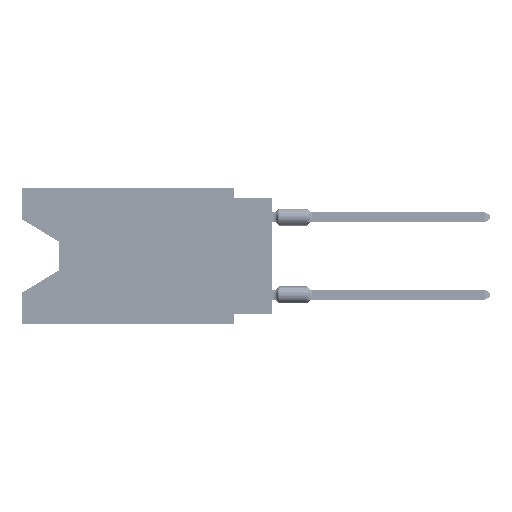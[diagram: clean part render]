
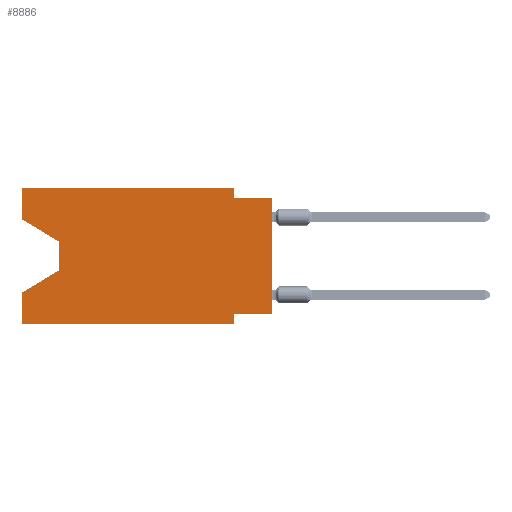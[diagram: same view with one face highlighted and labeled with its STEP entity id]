
A CAD part, left-side view. The second image highlights one B-rep face of the part: STEP entity #8886.
In plain terms, the highlighted planar face has unit normal (-1, 0, 0).
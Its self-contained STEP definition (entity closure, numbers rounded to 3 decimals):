
#264 = ORIENTED_EDGE ( 'NONE', *, *, #69302, .F. ) ;
#595 = CARTESIAN_POINT ( 'NONE',  ( 0., 13.97, -5.385 ) ) ;
#1083 = VERTEX_POINT ( 'NONE', #35631 ) ;
#1825 = VERTEX_POINT ( 'NONE', #34298 ) ;
#2641 = VERTEX_POINT ( 'NONE', #7301 ) ;
#3110 = LINE ( 'NONE', #29963, #32450 ) ;
#3960 = CARTESIAN_POINT ( 'NONE',  ( 0., 16.383, -6.852 ) ) ;
#4217 = CARTESIAN_POINT ( 'NONE',  ( 0., 16.383, 0. ) ) ;
#5352 = LINE ( 'NONE', #43268, #67273 ) ;
#5967 = LINE ( 'NONE', #595, #50175 ) ;
#7301 = CARTESIAN_POINT ( 'NONE',  ( 0., 2.54, 0. ) ) ;
#7393 = EDGE_CURVE ( 'NONE', #12482, #2641, #5352, .T. ) ;
#7450 = VERTEX_POINT ( 'NONE', #38617 ) ;
#7869 = VECTOR ( 'NONE', #42504, 1000. ) ;
#7970 = DIRECTION ( 'NONE',  ( 0., 1., 0. ) ) ;
#8477 = LINE ( 'NONE', #9177, #64732 ) ;
#8677 = DIRECTION ( 'NONE',  ( 0., 0., 1. ) ) ;
#8886 = ADVANCED_FACE ( 'NONE', ( #70002 ), #48882, .F. ) ;
#9177 = CARTESIAN_POINT ( 'NONE',  ( 0., 2.54, -8.89 ) ) ;
#10263 = DIRECTION ( 'NONE',  ( 1., 0., 0. ) ) ;
#11778 = DIRECTION ( 'NONE',  ( 0., 0., -1. ) ) ;
#11997 = CARTESIAN_POINT ( 'NONE',  ( 0., 13.97, -3.505 ) ) ;
#12122 = CARTESIAN_POINT ( 'NONE',  ( 0., 2.54, 0. ) ) ;
#12482 = VERTEX_POINT ( 'NONE', #26753 ) ;
#12996 = EDGE_CURVE ( 'NONE', #66328, #63262, #34804, .T. ) ;
#13418 = CARTESIAN_POINT ( 'NONE',  ( 0., 2.54, -8.89 ) ) ;
#13510 = EDGE_CURVE ( 'NONE', #26863, #36324, #62682, .T. ) ;
#14817 = LINE ( 'NONE', #36644, #32295 ) ;
#15714 = EDGE_CURVE ( 'NONE', #1825, #1083, #53208, .T. ) ;
#15821 = EDGE_CURVE ( 'NONE', #58953, #36324, #5967, .T. ) ;
#16925 = VERTEX_POINT ( 'NONE', #13418 ) ;
#19231 = CARTESIAN_POINT ( 'NONE',  ( 0., 0., -8.255 ) ) ;
#19946 = DIRECTION ( 'NONE',  ( 0., -0.855, -0.519 ) ) ;
#20306 = CARTESIAN_POINT ( 'NONE',  ( 0., 0., -0.635 ) ) ;
#20974 = ORIENTED_EDGE ( 'NONE', *, *, #15714, .F. ) ;
#21031 = DIRECTION ( 'NONE',  ( 0., -1., 0. ) ) ;
#21064 = ORIENTED_EDGE ( 'NONE', *, *, #13510, .F. ) ;
#23474 = DIRECTION ( 'NONE',  ( 0., 0.855, -0.519 ) ) ;
#23847 = LINE ( 'NONE', #44604, #47321 ) ;
#26753 = CARTESIAN_POINT ( 'NONE',  ( 0., 16.383, 0. ) ) ;
#26863 = VERTEX_POINT ( 'NONE', #33583 ) ;
#27519 = EDGE_CURVE ( 'NONE', #66328, #1083, #67367, .T. ) ;
#28102 = EDGE_CURVE ( 'NONE', #2641, #1825, #60772, .T. ) ;
#29053 = VECTOR ( 'NONE', #8677, 1000. ) ;
#29963 = CARTESIAN_POINT ( 'NONE',  ( 0., 16.383, -2.038 ) ) ;
#30712 = VECTOR ( 'NONE', #21031, 1000. ) ;
#30994 = DIRECTION ( 'NONE',  ( 0., 0., -1. ) ) ;
#32295 = VECTOR ( 'NONE', #57029, 1000. ) ;
#32450 = VECTOR ( 'NONE', #19946, 1000. ) ;
#32889 = DIRECTION ( 'NONE',  ( 0., -1., 0. ) ) ;
#33583 = CARTESIAN_POINT ( 'NONE',  ( 0., 16.383, -8.89 ) ) ;
#34298 = CARTESIAN_POINT ( 'NONE',  ( 0., 2.54, -0.635 ) ) ;
#34542 = ORIENTED_EDGE ( 'NONE', *, *, #56110, .T. ) ;
#34804 = LINE ( 'NONE', #67357, #57809 ) ;
#35147 = CARTESIAN_POINT ( 'NONE',  ( 0., 16.383, 0. ) ) ;
#35182 = ORIENTED_EDGE ( 'NONE', *, *, #7393, .F. ) ;
#35381 = ORIENTED_EDGE ( 'NONE', *, *, #15821, .T. ) ;
#35566 = ORIENTED_EDGE ( 'NONE', *, *, #43522, .T. ) ;
#35631 = CARTESIAN_POINT ( 'NONE',  ( 0., 0., -0.635 ) ) ;
#36324 = VERTEX_POINT ( 'NONE', #3960 ) ;
#36644 = CARTESIAN_POINT ( 'NONE',  ( 0., 16.383, -8.89 ) ) ;
#37811 = CARTESIAN_POINT ( 'NONE',  ( 0., 16.383, 0. ) ) ;
#38363 = CARTESIAN_POINT ( 'NONE',  ( 0., 2.54, -8.255 ) ) ;
#38617 = CARTESIAN_POINT ( 'NONE',  ( 0., 16.383, -2.038 ) ) ;
#40184 = DIRECTION ( 'NONE',  ( 0., 0., 1. ) ) ;
#40934 = VERTEX_POINT ( 'NONE', #11997 ) ;
#40956 = AXIS2_PLACEMENT_3D ( 'NONE', #37811, #10263, #42818 ) ;
#42504 = DIRECTION ( 'NONE',  ( 0., 0., 1. ) ) ;
#42818 = DIRECTION ( 'NONE',  ( 0., 0., -1. ) ) ;
#43268 = CARTESIAN_POINT ( 'NONE',  ( 0., 16.383, 0. ) ) ;
#43522 = EDGE_CURVE ( 'NONE', #7450, #40934, #3110, .T. ) ;
#44604 = CARTESIAN_POINT ( 'NONE',  ( 0., 13.97, -3.505 ) ) ;
#45418 = CARTESIAN_POINT ( 'NONE',  ( 0., 13.97, -5.385 ) ) ;
#46047 = VECTOR ( 'NONE', #11778, 1000. ) ;
#47321 = VECTOR ( 'NONE', #51034, 1000. ) ;
#48882 = PLANE ( 'NONE',  #40956 ) ;
#49479 = VECTOR ( 'NONE', #40184, 1000. ) ;
#50175 = VECTOR ( 'NONE', #23474, 1000. ) ;
#50234 = EDGE_CURVE ( 'NONE', #26863, #16925, #14817, .T. ) ;
#50338 = ORIENTED_EDGE ( 'NONE', *, *, #27519, .T. ) ;
#51034 = DIRECTION ( 'NONE',  ( 0., 0., -1. ) ) ;
#53208 = LINE ( 'NONE', #20306, #30712 ) ;
#54357 = ORIENTED_EDGE ( 'NONE', *, *, #12996, .F. ) ;
#54721 = ORIENTED_EDGE ( 'NONE', *, *, #50234, .T. ) ;
#55081 = ORIENTED_EDGE ( 'NONE', *, *, #58305, .F. ) ;
#55367 = EDGE_LOOP ( 'NONE', ( #35566, #34542, #35381, #21064, #54721, #55081, #54357, #50338, #20974, #65374, #35182, #264 ) ) ;
#56110 = EDGE_CURVE ( 'NONE', #40934, #58953, #23847, .T. ) ;
#57029 = DIRECTION ( 'NONE',  ( 0., -1., 0. ) ) ;
#57809 = VECTOR ( 'NONE', #7970, 1000. ) ;
#58305 = EDGE_CURVE ( 'NONE', #63262, #16925, #8477, .T. ) ;
#58944 = LINE ( 'NONE', #4217, #7869 ) ;
#58953 = VERTEX_POINT ( 'NONE', #45418 ) ;
#60772 = LINE ( 'NONE', #12122, #46047 ) ;
#62682 = LINE ( 'NONE', #35147, #29053 ) ;
#63262 = VERTEX_POINT ( 'NONE', #38363 ) ;
#64732 = VECTOR ( 'NONE', #30994, 1000. ) ;
#65374 = ORIENTED_EDGE ( 'NONE', *, *, #28102, .F. ) ;
#66328 = VERTEX_POINT ( 'NONE', #19231 ) ;
#67273 = VECTOR ( 'NONE', #32889, 1000. ) ;
#67357 = CARTESIAN_POINT ( 'NONE',  ( 0., 0., -8.255 ) ) ;
#67367 = LINE ( 'NONE', #67730, #49479 ) ;
#67730 = CARTESIAN_POINT ( 'NONE',  ( 0., 0., 0. ) ) ;
#69302 = EDGE_CURVE ( 'NONE', #7450, #12482, #58944, .T. ) ;
#70002 = FACE_OUTER_BOUND ( 'NONE', #55367, .T. ) ;
